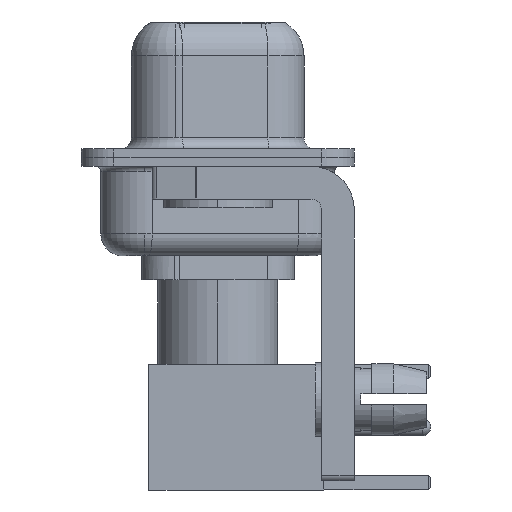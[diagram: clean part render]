
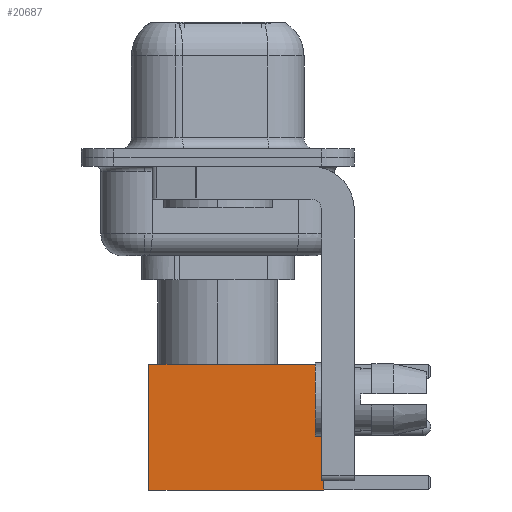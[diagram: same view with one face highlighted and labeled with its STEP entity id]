
A CAD part, left-side view. The second image highlights one B-rep face of the part: STEP entity #20687.
In plain terms, the highlighted face is planar.
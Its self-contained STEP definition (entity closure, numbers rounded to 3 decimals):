
#22 = LINE ( 'NONE', #6415, #17269 ) ;
#1934 = FACE_OUTER_BOUND ( 'NONE', #6254, .T. ) ;
#2105 = CARTESIAN_POINT ( 'NONE',  ( 2.875, 2.875, 0. ) ) ;
#2831 = ORIENTED_EDGE ( 'NONE', *, *, #17773, .F. ) ;
#2834 = AXIS2_PLACEMENT_3D ( 'NONE', #8346, #12665, #12969 ) ;
#3551 = DIRECTION ( 'NONE',  ( -1., 0., 0. ) ) ;
#3719 = DIRECTION ( 'NONE',  ( 0., 0., -1. ) ) ;
#4527 = DIRECTION ( 'NONE',  ( -1., 0., 0. ) ) ;
#4530 = VECTOR ( 'NONE', #3719, 1000. ) ;
#4695 = CARTESIAN_POINT ( 'NONE',  ( -2.875, 2.875, 8. ) ) ;
#4755 = PLANE ( 'NONE',  #2834 ) ;
#5292 = LINE ( 'NONE', #11707, #4530 ) ;
#5551 = VECTOR ( 'NONE', #4527, 1000. ) ;
#6254 = EDGE_LOOP ( 'NONE', ( #6345, #15491, #15839, #2831 ) ) ;
#6345 = ORIENTED_EDGE ( 'NONE', *, *, #13667, .T. ) ;
#6415 = CARTESIAN_POINT ( 'NONE',  ( -2.875, 2.875, 0. ) ) ;
#7572 = EDGE_CURVE ( 'NONE', #12696, #16977, #22, .T. ) ;
#8053 = LINE ( 'NONE', #8382, #10794 ) ;
#8346 = CARTESIAN_POINT ( 'NONE',  ( 2.875, 2.875, 0. ) ) ;
#8382 = CARTESIAN_POINT ( 'NONE',  ( 0., 2.875, 8. ) ) ;
#10794 = VECTOR ( 'NONE', #3551, 1000. ) ;
#11605 = VERTEX_POINT ( 'NONE', #20022 ) ;
#11707 = CARTESIAN_POINT ( 'NONE',  ( 2.875, 2.875, 0. ) ) ;
#12082 = EDGE_CURVE ( 'NONE', #12349, #16977, #20500, .T. ) ;
#12349 = VERTEX_POINT ( 'NONE', #2105 ) ;
#12665 = DIRECTION ( 'NONE',  ( 0., 1., 0. ) ) ;
#12696 = VERTEX_POINT ( 'NONE', #4695 ) ;
#12969 = DIRECTION ( 'NONE',  ( 0., 0., 1. ) ) ;
#13667 = EDGE_CURVE ( 'NONE', #11605, #12349, #5292, .T. ) ;
#15491 = ORIENTED_EDGE ( 'NONE', *, *, #12082, .T. ) ;
#15839 = ORIENTED_EDGE ( 'NONE', *, *, #7572, .F. ) ;
#16977 = VERTEX_POINT ( 'NONE', #18017 ) ;
#17269 = VECTOR ( 'NONE', #19260, 1000. ) ;
#17773 = EDGE_CURVE ( 'NONE', #11605, #12696, #8053, .T. ) ;
#18017 = CARTESIAN_POINT ( 'NONE',  ( -2.875, 2.875, 0. ) ) ;
#18924 = CARTESIAN_POINT ( 'NONE',  ( 0., 2.875, 0. ) ) ;
#19260 = DIRECTION ( 'NONE',  ( 0., 0., -1. ) ) ;
#20022 = CARTESIAN_POINT ( 'NONE',  ( 2.875, 2.875, 8. ) ) ;
#20500 = LINE ( 'NONE', #18924, #5551 ) ;
#20687 = ADVANCED_FACE ( 'NONE', ( #1934 ), #4755, .T. ) ;
